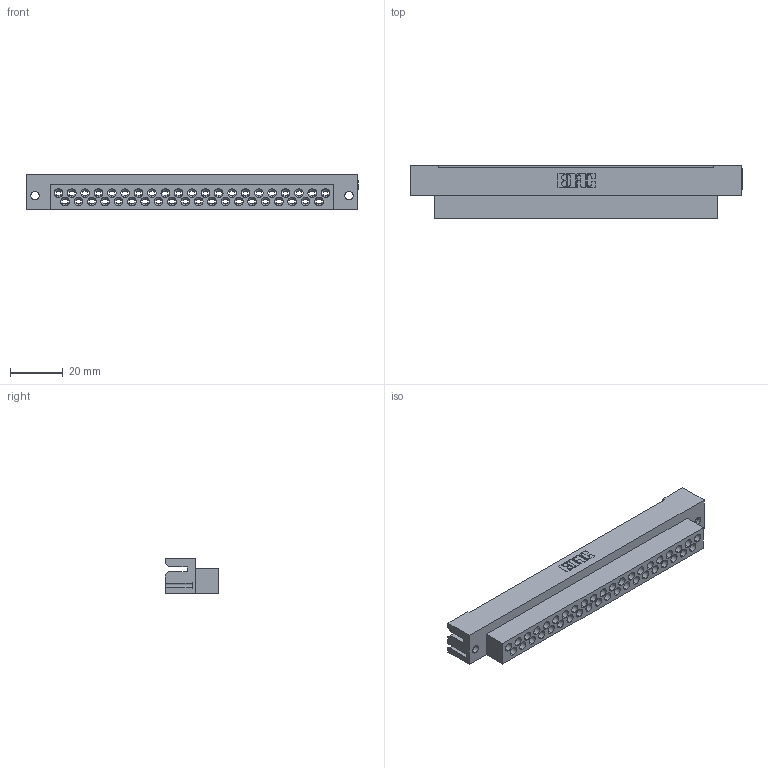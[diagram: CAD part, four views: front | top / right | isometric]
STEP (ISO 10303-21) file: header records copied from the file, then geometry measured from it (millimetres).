
FILE_DESCRIPTION (( 'STEP AP203' ), '1' );
FILE_NAME ('438-041-000-112.STEP', '2020-03-12T20:54:40', ( '' ), ( '' ), 'SwSTEP 2.0', 'SolidWorks 2016', '' );
FILE_SCHEMA (( 'CONFIG_CONTROL_DESIGN' ));
Length unit declared in the file: millimetre
Products named in the file (2): 438-210-001_438-210-041-112; 438-041-000-112
Assembly tree (1 placements, depth 2):
  438-041-000-112
    438-210-001_438-210-041-112
Bounding box: 126.24 x 20.45 x 13.49 mm (x, y, z)
Volume: 19529.7 mm3; surface area: 19446.6 mm2
Topology: 1 solids, 1 shells, 1214 faces, 3616 edges, 2369 vertices
Faces by surface type: plane 937, cylinder 132, cone 123, bspline 22
Entity records: 42049 total; most frequent: CARTESIAN_POINT 9765, ORIENTED_EDGE 7232, DIRECTION 6029, EDGE_CURVE 3616, LINE 2523, VECTOR 2523, VERTEX_POINT 2369, AXIS2_PLACEMENT_3D 1753
